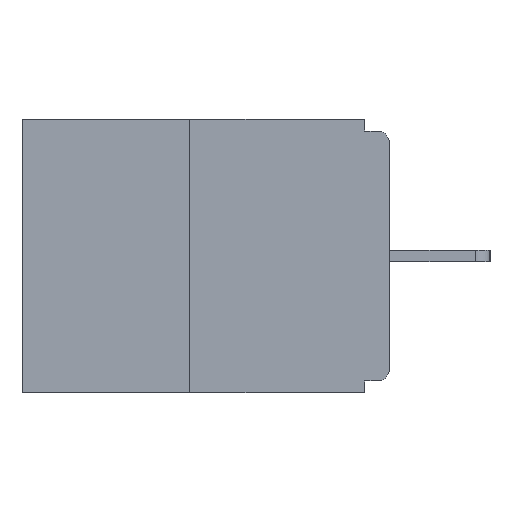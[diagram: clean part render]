
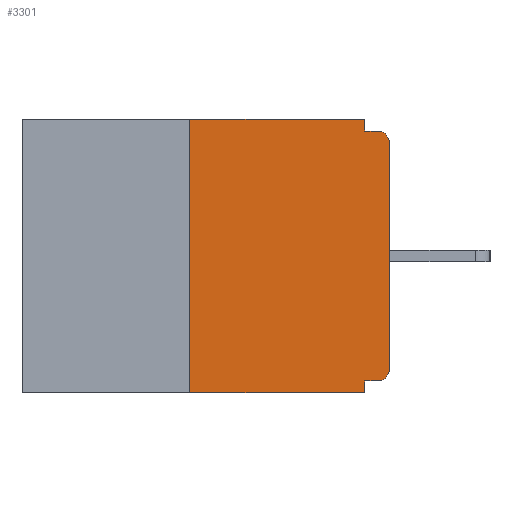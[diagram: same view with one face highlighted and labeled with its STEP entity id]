
A CAD part, left-side view. The second image highlights one B-rep face of the part: STEP entity #3301.
In plain terms, the highlighted planar face has unit normal (-1, 0, 0).
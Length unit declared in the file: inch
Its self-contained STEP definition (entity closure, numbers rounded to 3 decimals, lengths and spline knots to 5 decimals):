
#85 = CARTESIAN_POINT ( 'NONE',  ( 0., 0.015, -0.03 ) ) ;
#445 = VECTOR ( 'NONE', #13036, 39.37008 ) ;
#468 = EDGE_CURVE ( 'NONE', #21214, #4056, #6591, .T. ) ;
#1261 = CARTESIAN_POINT ( 'NONE',  ( 0., 0., -0.015 ) ) ;
#1345 = EDGE_CURVE ( 'NONE', #2204, #21707, #22598, .T. ) ;
#1491 = AXIS2_PLACEMENT_3D ( 'NONE', #15380, #6652, #22597 ) ;
#2204 = VERTEX_POINT ( 'NONE', #19675 ) ;
#2258 = ORIENTED_EDGE ( 'NONE', *, *, #2290, .F. ) ;
#2290 = EDGE_CURVE ( 'NONE', #2738, #15110, #20366, .T. ) ;
#2615 = CARTESIAN_POINT ( 'NONE',  ( 0., 0.031, -0.343 ) ) ;
#2738 = VERTEX_POINT ( 'NONE', #10449 ) ;
#3055 = LINE ( 'NONE', #3170, #10848 ) ;
#3102 = EDGE_CURVE ( 'NONE', #4488, #21707, #18735, .T. ) ;
#3170 = CARTESIAN_POINT ( 'NONE',  ( 0., 0., -0.328 ) ) ;
#3186 = DIRECTION ( 'NONE',  ( 0., 0., 1. ) ) ;
#3246 = CARTESIAN_POINT ( 'NONE',  ( 0., 0.031, -0.343 ) ) ;
#3301 = ADVANCED_FACE ( 'NONE', ( #6977 ), #10530, .F. ) ;
#3390 = ORIENTED_EDGE ( 'NONE', *, *, #17955, .T. ) ;
#3516 = ORIENTED_EDGE ( 'NONE', *, *, #7079, .F. ) ;
#4056 = VERTEX_POINT ( 'NONE', #6557 ) ;
#4213 = LINE ( 'NONE', #18165, #6053 ) ;
#4488 = VERTEX_POINT ( 'NONE', #15565 ) ;
#4749 = CARTESIAN_POINT ( 'NONE',  ( 0., 0.46, 0. ) ) ;
#5271 = DIRECTION ( 'NONE',  ( 0., 0., -1. ) ) ;
#5326 = DIRECTION ( 'NONE',  ( 0., 0., -1. ) ) ;
#5540 = DIRECTION ( 'NONE',  ( 0., 0., -1. ) ) ;
#5660 = EDGE_CURVE ( 'NONE', #4056, #11228, #6918, .T. ) ;
#6053 = VECTOR ( 'NONE', #5540, 39.37008 ) ;
#6217 = LINE ( 'NONE', #4749, #13122 ) ;
#6557 = CARTESIAN_POINT ( 'NONE',  ( 0., 0., -0.313 ) ) ;
#6568 = ORIENTED_EDGE ( 'NONE', *, *, #12971, .F. ) ;
#6591 = CIRCLE ( 'NONE', #1491, 0.015 ) ;
#6652 = DIRECTION ( 'NONE',  ( -1., 0., 0. ) ) ;
#6918 = LINE ( 'NONE', #10470, #19482 ) ;
#6977 = FACE_OUTER_BOUND ( 'NONE', #14588, .T. ) ;
#7079 = EDGE_CURVE ( 'NONE', #12000, #2738, #4213, .T. ) ;
#8043 = ORIENTED_EDGE ( 'NONE', *, *, #15010, .F. ) ;
#8382 = DIRECTION ( 'NONE',  ( 0., -1., 0. ) ) ;
#9587 = VECTOR ( 'NONE', #8382, 39.37008 ) ;
#10271 = CARTESIAN_POINT ( 'NONE',  ( 0., 0., -0.03 ) ) ;
#10449 = CARTESIAN_POINT ( 'NONE',  ( 0., 0.031, -0.015 ) ) ;
#10470 = CARTESIAN_POINT ( 'NONE',  ( 0., 0., 0. ) ) ;
#10530 = PLANE ( 'NONE',  #18053 ) ;
#10848 = VECTOR ( 'NONE', #15636, 39.37008 ) ;
#11228 = VERTEX_POINT ( 'NONE', #10271 ) ;
#12000 = VERTEX_POINT ( 'NONE', #13535 ) ;
#12303 = ORIENTED_EDGE ( 'NONE', *, *, #5660, .T. ) ;
#12524 = AXIS2_PLACEMENT_3D ( 'NONE', #85, #17500, #5326 ) ;
#12971 = EDGE_CURVE ( 'NONE', #21214, #2204, #3055, .T. ) ;
#13036 = DIRECTION ( 'NONE',  ( 0., -1., 0. ) ) ;
#13122 = VECTOR ( 'NONE', #18841, 39.37008 ) ;
#13466 = ORIENTED_EDGE ( 'NONE', *, *, #19886, .F. ) ;
#13535 = CARTESIAN_POINT ( 'NONE',  ( 0., 0.031, 0. ) ) ;
#13574 = CARTESIAN_POINT ( 'NONE',  ( 0., 0.46, -0.343 ) ) ;
#13886 = CARTESIAN_POINT ( 'NONE',  ( 0., 0.25, 0. ) ) ;
#13993 = DIRECTION ( 'NONE',  ( 1., 0., 0. ) ) ;
#14588 = EDGE_LOOP ( 'NONE', ( #13466, #8043, #21487, #15147, #6568, #22070, #12303, #3390, #2258, #3516 ) ) ;
#14738 = CIRCLE ( 'NONE', #12524, 0.015 ) ;
#15010 = EDGE_CURVE ( 'NONE', #4488, #16887, #18579, .T. ) ;
#15110 = VERTEX_POINT ( 'NONE', #21316 ) ;
#15147 = ORIENTED_EDGE ( 'NONE', *, *, #1345, .F. ) ;
#15153 = CARTESIAN_POINT ( 'NONE',  ( 0., 0.25, 0. ) ) ;
#15380 = CARTESIAN_POINT ( 'NONE',  ( 0., 0.015, -0.313 ) ) ;
#15565 = CARTESIAN_POINT ( 'NONE',  ( 0., 0.25, -0.343 ) ) ;
#15636 = DIRECTION ( 'NONE',  ( 0., 1., 0. ) ) ;
#15685 = VECTOR ( 'NONE', #22360, 39.37008 ) ;
#16887 = VERTEX_POINT ( 'NONE', #13886 ) ;
#16992 = DIRECTION ( 'NONE',  ( 0., 0., -1. ) ) ;
#17331 = CARTESIAN_POINT ( 'NONE',  ( 0., 0.46, 0. ) ) ;
#17500 = DIRECTION ( 'NONE',  ( -1., 0., 0. ) ) ;
#17955 = EDGE_CURVE ( 'NONE', #11228, #15110, #14738, .T. ) ;
#18053 = AXIS2_PLACEMENT_3D ( 'NONE', #17331, #13993, #5271 ) ;
#18165 = CARTESIAN_POINT ( 'NONE',  ( 0., 0.031, 0. ) ) ;
#18579 = LINE ( 'NONE', #15153, #15685 ) ;
#18735 = LINE ( 'NONE', #13574, #9587 ) ;
#18841 = DIRECTION ( 'NONE',  ( 0., -1., 0. ) ) ;
#19482 = VECTOR ( 'NONE', #3186, 39.37008 ) ;
#19675 = CARTESIAN_POINT ( 'NONE',  ( 0., 0.031, -0.328 ) ) ;
#19817 = VECTOR ( 'NONE', #16992, 39.37008 ) ;
#19886 = EDGE_CURVE ( 'NONE', #16887, #12000, #6217, .T. ) ;
#20366 = LINE ( 'NONE', #1261, #445 ) ;
#21214 = VERTEX_POINT ( 'NONE', #21804 ) ;
#21316 = CARTESIAN_POINT ( 'NONE',  ( 0., 0.015, -0.015 ) ) ;
#21487 = ORIENTED_EDGE ( 'NONE', *, *, #3102, .T. ) ;
#21707 = VERTEX_POINT ( 'NONE', #2615 ) ;
#21804 = CARTESIAN_POINT ( 'NONE',  ( 0., 0.015, -0.328 ) ) ;
#22070 = ORIENTED_EDGE ( 'NONE', *, *, #468, .T. ) ;
#22360 = DIRECTION ( 'NONE',  ( 0., 0., 1. ) ) ;
#22597 = DIRECTION ( 'NONE',  ( 0., 0., -1. ) ) ;
#22598 = LINE ( 'NONE', #3246, #19817 ) ;
